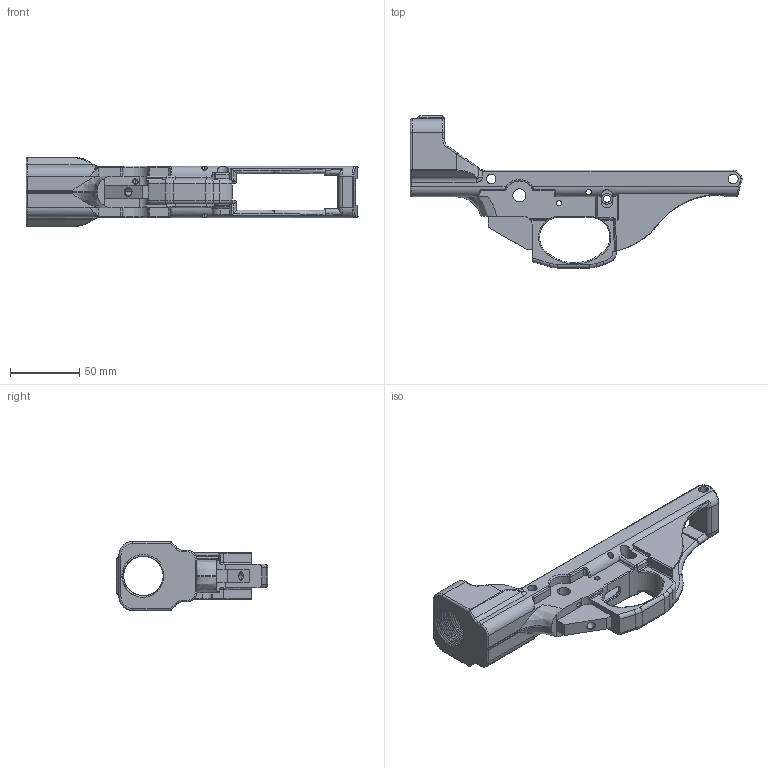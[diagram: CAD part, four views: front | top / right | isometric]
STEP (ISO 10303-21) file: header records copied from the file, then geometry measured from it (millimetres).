
FILE_DESCRIPTION (( 'STEP AP214' ), '1' );
FILE_NAME ('Caleb_AR-10_V1.STEP', '2015-05-21T10:24:22', ( 'WarFairy' ), ( '' ), 'SwSTEP 2.0', 'SolidWorks 2015', '' );
FILE_SCHEMA (( 'AUTOMOTIVE_DESIGN' ));
Length unit declared in the file: millimetre
Products named in the file (1): Caleb_AR-10_V1
Bounding box: 239.65 x 109.71 x 50 mm (x, y, z)
Volume: 178666.3 mm3; surface area: 59264.4 mm2
Topology: 1 solids, 5 shells, 489 faces, 1317 edges, 817 vertices
Faces by surface type: cylinder 219, plane 116, bspline 97, torus 51, sphere 4, cone 2
Entity records: 34719 total; most frequent: CARTESIAN_POINT 20345, ORIENTED_EDGE 2606, DIRECTION 2092, EDGE_CURVE 1303, VERTEX_POINT 817, AXIS2_PLACEMENT_3D 799, EDGE_LOOP 518, VECTOR 494
